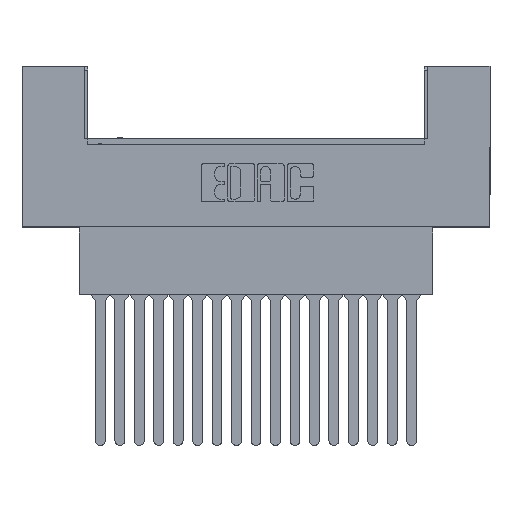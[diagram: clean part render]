
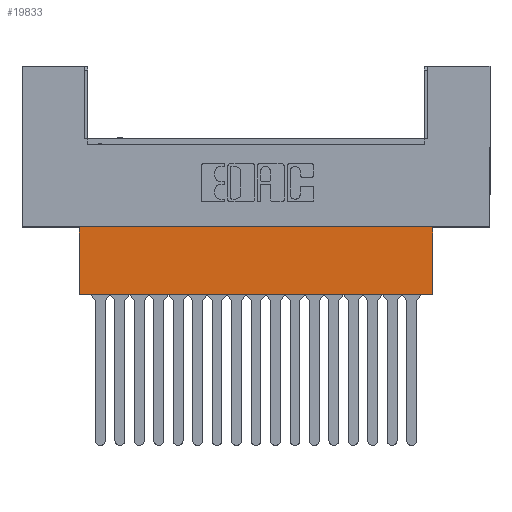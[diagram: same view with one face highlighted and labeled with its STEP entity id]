
A CAD part, top view. The second image highlights one B-rep face of the part: STEP entity #19833.
In plain terms, the highlighted planar face has unit normal (0, 0, 1).
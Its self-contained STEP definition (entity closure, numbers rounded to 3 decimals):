
#761 = VERTEX_POINT ( 'NONE', #23865 ) ;
#841 = EDGE_CURVE ( 'NONE', #761, #15072, #9952, .T. ) ;
#902 = CARTESIAN_POINT ( 'NONE',  ( 61.112, 0., -3.962 ) ) ;
#1249 = LINE ( 'NONE', #902, #8876 ) ;
#2021 = CARTESIAN_POINT ( 'NONE',  ( 7.468, 0., -3.962 ) ) ;
#3206 = DIRECTION ( 'NONE',  ( 0., 0., -1. ) ) ;
#5180 = DIRECTION ( 'NONE',  ( 0., 1., 0. ) ) ;
#6850 = VECTOR ( 'NONE', #19356, 1000. ) ;
#7745 = LINE ( 'NONE', #23072, #6850 ) ;
#8563 = DIRECTION ( 'NONE',  ( -1., 0., 0. ) ) ;
#8707 = ORIENTED_EDGE ( 'NONE', *, *, #12617, .T. ) ;
#8876 = VECTOR ( 'NONE', #21273, 1000. ) ;
#9233 = VERTEX_POINT ( 'NONE', #17752 ) ;
#9952 = LINE ( 'NONE', #18551, #21415 ) ;
#10336 = ORIENTED_EDGE ( 'NONE', *, *, #841, .F. ) ;
#11394 = VERTEX_POINT ( 'NONE', #23971 ) ;
#11742 = FACE_OUTER_BOUND ( 'NONE', #23361, .T. ) ;
#11881 = EDGE_CURVE ( 'NONE', #11394, #761, #17110, .T. ) ;
#12425 = VECTOR ( 'NONE', #8563, 1000. ) ;
#12617 = EDGE_CURVE ( 'NONE', #9233, #15072, #1249, .T. ) ;
#14448 = ORIENTED_EDGE ( 'NONE', *, *, #11881, .F. ) ;
#15072 = VERTEX_POINT ( 'NONE', #2021 ) ;
#17110 = LINE ( 'NONE', #19907, #12425 ) ;
#17692 = AXIS2_PLACEMENT_3D ( 'NONE', #18308, #3206, #20141 ) ;
#17752 = CARTESIAN_POINT ( 'NONE',  ( 53.645, 0., -3.962 ) ) ;
#18308 = CARTESIAN_POINT ( 'NONE',  ( 61.112, 0., -3.962 ) ) ;
#18551 = CARTESIAN_POINT ( 'NONE',  ( 7.468, -8.814, -3.962 ) ) ;
#19356 = DIRECTION ( 'NONE',  ( 0., -1., 0. ) ) ;
#19833 = ADVANCED_FACE ( 'NONE', ( #11742 ), #23695, .F. ) ;
#19907 = CARTESIAN_POINT ( 'NONE',  ( 61.112, -8.814, -3.962 ) ) ;
#20141 = DIRECTION ( 'NONE',  ( 0., 1., 0. ) ) ;
#20953 = ORIENTED_EDGE ( 'NONE', *, *, #24340, .F. ) ;
#21273 = DIRECTION ( 'NONE',  ( -1., 0., 0. ) ) ;
#21415 = VECTOR ( 'NONE', #5180, 1000. ) ;
#23072 = CARTESIAN_POINT ( 'NONE',  ( 53.645, -8.814, -3.962 ) ) ;
#23361 = EDGE_LOOP ( 'NONE', ( #14448, #20953, #8707, #10336 ) ) ;
#23695 = PLANE ( 'NONE',  #17692 ) ;
#23865 = CARTESIAN_POINT ( 'NONE',  ( 7.468, -8.814, -3.962 ) ) ;
#23971 = CARTESIAN_POINT ( 'NONE',  ( 53.645, -8.814, -3.962 ) ) ;
#24340 = EDGE_CURVE ( 'NONE', #9233, #11394, #7745, .T. ) ;
